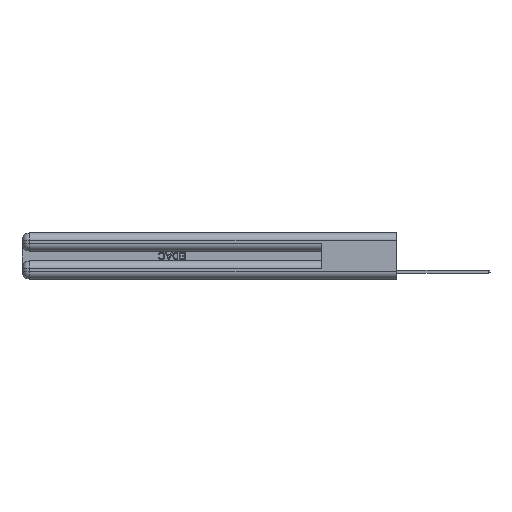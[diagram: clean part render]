
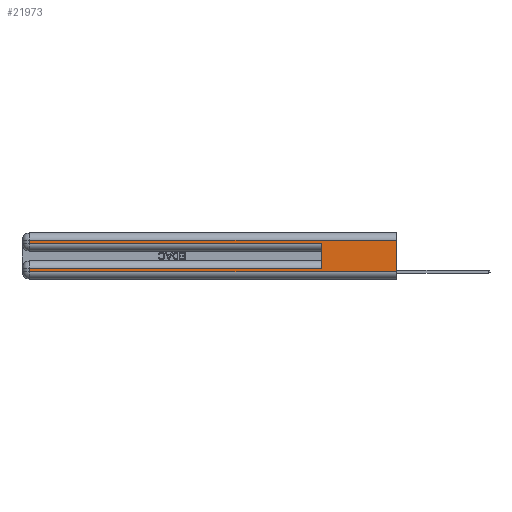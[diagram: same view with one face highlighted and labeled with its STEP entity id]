
A CAD part, left-side view. The second image highlights one B-rep face of the part: STEP entity #21973.
In plain terms, the highlighted planar face has unit normal (-1, 0, 0).
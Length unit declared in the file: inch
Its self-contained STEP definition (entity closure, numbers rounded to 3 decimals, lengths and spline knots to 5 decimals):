
#123 = CARTESIAN_POINT ( 'NONE',  ( 0., 0., 0.37 ) ) ;
#395 = DIRECTION ( 'NONE',  ( 0., 0., -1. ) ) ;
#450 = VECTOR ( 'NONE', #19334, 39.37008 ) ;
#475 = ORIENTED_EDGE ( 'NONE', *, *, #7531, .T. ) ;
#2809 = CARTESIAN_POINT ( 'NONE',  ( 0., 0., 0.31 ) ) ;
#5354 = CARTESIAN_POINT ( 'NONE',  ( 0., 0., 0.085 ) ) ;
#5545 = LINE ( 'NONE', #16035, #12114 ) ;
#6489 = EDGE_CURVE ( 'NONE', #30700, #9666, #28114, .T. ) ;
#6794 = CARTESIAN_POINT ( 'NONE',  ( 0., 2.94, 0.06 ) ) ;
#6811 = VERTEX_POINT ( 'NONE', #6794 ) ;
#7531 = EDGE_CURVE ( 'NONE', #14689, #17157, #31694, .T. ) ;
#8128 = LINE ( 'NONE', #22333, #15508 ) ;
#8314 = LINE ( 'NONE', #123, #16958 ) ;
#8785 = DIRECTION ( 'NONE',  ( 1., 0., 0. ) ) ;
#8794 = EDGE_LOOP ( 'NONE', ( #32056, #16997, #28611, #27252, #13741, #475, #24514, #19690 ) ) ;
#8897 = CARTESIAN_POINT ( 'NONE',  ( 0., 0., 0.37 ) ) ;
#9351 = DIRECTION ( 'NONE',  ( 0., -1., 0. ) ) ;
#9666 = VERTEX_POINT ( 'NONE', #17372 ) ;
#11732 = EDGE_CURVE ( 'NONE', #30700, #15884, #8314, .T. ) ;
#12114 = VECTOR ( 'NONE', #395, 39.37008 ) ;
#12204 = EDGE_CURVE ( 'NONE', #17157, #6811, #25057, .T. ) ;
#13741 = ORIENTED_EDGE ( 'NONE', *, *, #18985, .F. ) ;
#13847 = PLANE ( 'NONE',  #27923 ) ;
#14689 = VERTEX_POINT ( 'NONE', #19691 ) ;
#15330 = LINE ( 'NONE', #28633, #29524 ) ;
#15508 = VECTOR ( 'NONE', #9351, 39.37008 ) ;
#15814 = DIRECTION ( 'NONE',  ( 0., -1., 0. ) ) ;
#15822 = VERTEX_POINT ( 'NONE', #23616 ) ;
#15884 = VERTEX_POINT ( 'NONE', #30014 ) ;
#16035 = CARTESIAN_POINT ( 'NONE',  ( 0., 2.94, 0.37 ) ) ;
#16958 = VECTOR ( 'NONE', #18711, 39.37008 ) ;
#16997 = ORIENTED_EDGE ( 'NONE', *, *, #6489, .T. ) ;
#17157 = VERTEX_POINT ( 'NONE', #19329 ) ;
#17372 = CARTESIAN_POINT ( 'NONE',  ( 0., 2.94, 0.31 ) ) ;
#18039 = EDGE_CURVE ( 'NONE', #6811, #15884, #8128, .T. ) ;
#18376 = DIRECTION ( 'NONE',  ( 0., 1., 0. ) ) ;
#18548 = CARTESIAN_POINT ( 'NONE',  ( 0., 0., 0.31 ) ) ;
#18711 = DIRECTION ( 'NONE',  ( 0., 0., -1. ) ) ;
#18985 = EDGE_CURVE ( 'NONE', #14689, #15822, #26515, .T. ) ;
#19329 = CARTESIAN_POINT ( 'NONE',  ( 0., 2.94, 0.085 ) ) ;
#19334 = DIRECTION ( 'NONE',  ( 0., 0., 1. ) ) ;
#19690 = ORIENTED_EDGE ( 'NONE', *, *, #18039, .T. ) ;
#19691 = CARTESIAN_POINT ( 'NONE',  ( 0., 0.6, 0.085 ) ) ;
#20421 = VERTEX_POINT ( 'NONE', #20829 ) ;
#20829 = CARTESIAN_POINT ( 'NONE',  ( 0., 2.94, 0.285 ) ) ;
#21496 = CARTESIAN_POINT ( 'NONE',  ( 0., 0.6, 0.145 ) ) ;
#21797 = VECTOR ( 'NONE', #30358, 39.37008 ) ;
#21973 = ADVANCED_FACE ( 'NONE', ( #30033 ), #13847, .F. ) ;
#22333 = CARTESIAN_POINT ( 'NONE',  ( 0., 0., 0.06 ) ) ;
#22405 = EDGE_CURVE ( 'NONE', #9666, #20421, #5545, .T. ) ;
#23616 = CARTESIAN_POINT ( 'NONE',  ( 0., 0.6, 0.285 ) ) ;
#24514 = ORIENTED_EDGE ( 'NONE', *, *, #12204, .T. ) ;
#24673 = DIRECTION ( 'NONE',  ( 0., 1., 0. ) ) ;
#25057 = LINE ( 'NONE', #27642, #21797 ) ;
#26515 = LINE ( 'NONE', #21496, #450 ) ;
#26777 = DIRECTION ( 'NONE',  ( 0., 0., -1. ) ) ;
#27252 = ORIENTED_EDGE ( 'NONE', *, *, #29413, .T. ) ;
#27642 = CARTESIAN_POINT ( 'NONE',  ( 0., 2.94, 0.37 ) ) ;
#27923 = AXIS2_PLACEMENT_3D ( 'NONE', #8897, #8785, #26777 ) ;
#28090 = VECTOR ( 'NONE', #18376, 39.37008 ) ;
#28114 = LINE ( 'NONE', #18548, #30125 ) ;
#28611 = ORIENTED_EDGE ( 'NONE', *, *, #22405, .T. ) ;
#28633 = CARTESIAN_POINT ( 'NONE',  ( 0., 0., 0.285 ) ) ;
#29413 = EDGE_CURVE ( 'NONE', #20421, #15822, #15330, .T. ) ;
#29524 = VECTOR ( 'NONE', #15814, 39.37008 ) ;
#30014 = CARTESIAN_POINT ( 'NONE',  ( 0., 0., 0.06 ) ) ;
#30033 = FACE_OUTER_BOUND ( 'NONE', #8794, .T. ) ;
#30125 = VECTOR ( 'NONE', #24673, 39.37008 ) ;
#30358 = DIRECTION ( 'NONE',  ( 0., 0., -1. ) ) ;
#30700 = VERTEX_POINT ( 'NONE', #2809 ) ;
#31694 = LINE ( 'NONE', #5354, #28090 ) ;
#32056 = ORIENTED_EDGE ( 'NONE', *, *, #11732, .F. ) ;
